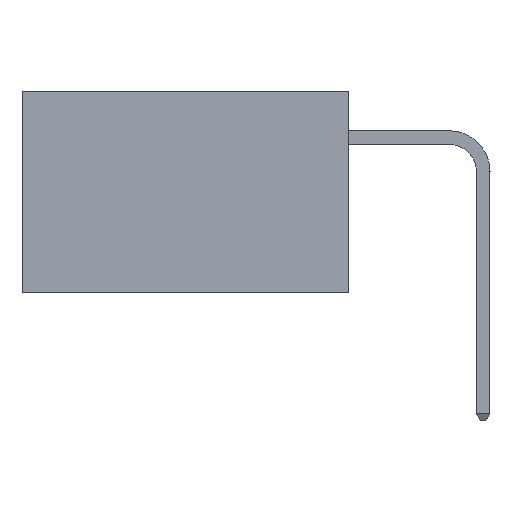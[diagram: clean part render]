
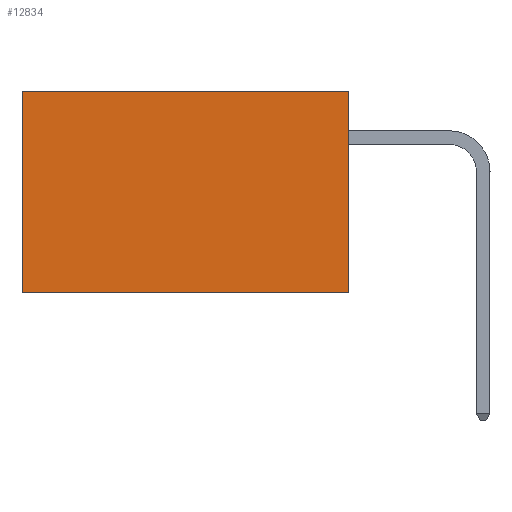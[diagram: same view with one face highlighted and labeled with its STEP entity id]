
A CAD part, left-side view. The second image highlights one B-rep face of the part: STEP entity #12834.
In plain terms, the highlighted planar face has unit normal (-1, 0, 0).
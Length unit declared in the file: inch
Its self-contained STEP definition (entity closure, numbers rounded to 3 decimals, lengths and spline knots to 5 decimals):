
#265 = LINE ( 'NONE', #5699, #7935 ) ;
#1793 = EDGE_CURVE ( 'NONE', #1833, #17677, #15715, .T. ) ;
#1833 = VERTEX_POINT ( 'NONE', #1927 ) ;
#1927 = CARTESIAN_POINT ( 'NONE',  ( 0.2875, 0., -0.37 ) ) ;
#2885 = EDGE_CURVE ( 'NONE', #3189, #1833, #265, .T. ) ;
#3189 = VERTEX_POINT ( 'NONE', #4747 ) ;
#4267 = VECTOR ( 'NONE', #15478, 39.37008 ) ;
#4700 = DIRECTION ( 'NONE',  ( 0., 1., 0. ) ) ;
#4747 = CARTESIAN_POINT ( 'NONE',  ( 0.2875, 0., 0. ) ) ;
#4777 = CARTESIAN_POINT ( 'NONE',  ( 0.2875, 0., -0.37 ) ) ;
#5699 = CARTESIAN_POINT ( 'NONE',  ( 0.2875, 0., 0. ) ) ;
#5826 = VECTOR ( 'NONE', #9693, 39.37008 ) ;
#7070 = EDGE_CURVE ( 'NONE', #3189, #8631, #13362, .T. ) ;
#7210 = EDGE_LOOP ( 'NONE', ( #14253, #15394, #10051, #8275 ) ) ;
#7253 = CARTESIAN_POINT ( 'NONE',  ( 0.2875, 0.6, 0. ) ) ;
#7265 = DIRECTION ( 'NONE',  ( 1., 0., 0. ) ) ;
#7935 = VECTOR ( 'NONE', #11219, 39.37008 ) ;
#8275 = ORIENTED_EDGE ( 'NONE', *, *, #7070, .T. ) ;
#8631 = VERTEX_POINT ( 'NONE', #7253 ) ;
#9693 = DIRECTION ( 'NONE',  ( 0., 1., 0. ) ) ;
#9755 = CARTESIAN_POINT ( 'NONE',  ( 0.2875, 0., 0. ) ) ;
#10051 = ORIENTED_EDGE ( 'NONE', *, *, #2885, .F. ) ;
#11219 = DIRECTION ( 'NONE',  ( 0., 0., -1. ) ) ;
#11554 = VECTOR ( 'NONE', #4700, 39.37008 ) ;
#12222 = CARTESIAN_POINT ( 'NONE',  ( 0.2875, 0.6, -0.37 ) ) ;
#12834 = ADVANCED_FACE ( 'NONE', ( #12849 ), #17064, .F. ) ;
#12849 = FACE_OUTER_BOUND ( 'NONE', #7210, .T. ) ;
#13362 = LINE ( 'NONE', #9755, #5826 ) ;
#14253 = ORIENTED_EDGE ( 'NONE', *, *, #17301, .T. ) ;
#15112 = LINE ( 'NONE', #18237, #4267 ) ;
#15394 = ORIENTED_EDGE ( 'NONE', *, *, #1793, .F. ) ;
#15478 = DIRECTION ( 'NONE',  ( 0., 0., -1. ) ) ;
#15715 = LINE ( 'NONE', #4777, #11554 ) ;
#15716 = CARTESIAN_POINT ( 'NONE',  ( 0.2875, 0., 0. ) ) ;
#17064 = PLANE ( 'NONE',  #17788 ) ;
#17121 = DIRECTION ( 'NONE',  ( 0., 0., -1. ) ) ;
#17301 = EDGE_CURVE ( 'NONE', #8631, #17677, #15112, .T. ) ;
#17677 = VERTEX_POINT ( 'NONE', #12222 ) ;
#17788 = AXIS2_PLACEMENT_3D ( 'NONE', #15716, #7265, #17121 ) ;
#18237 = CARTESIAN_POINT ( 'NONE',  ( 0.2875, 0.6, 0. ) ) ;
